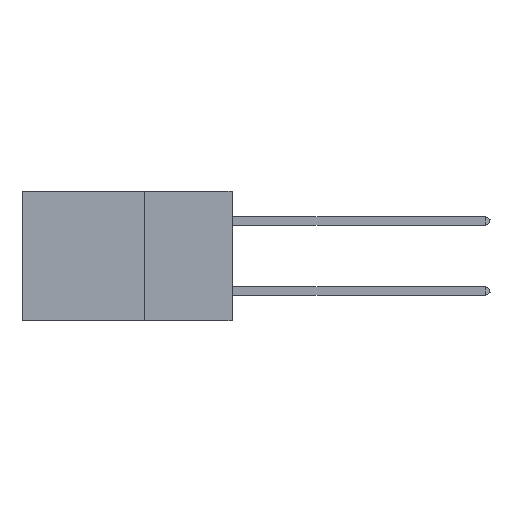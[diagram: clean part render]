
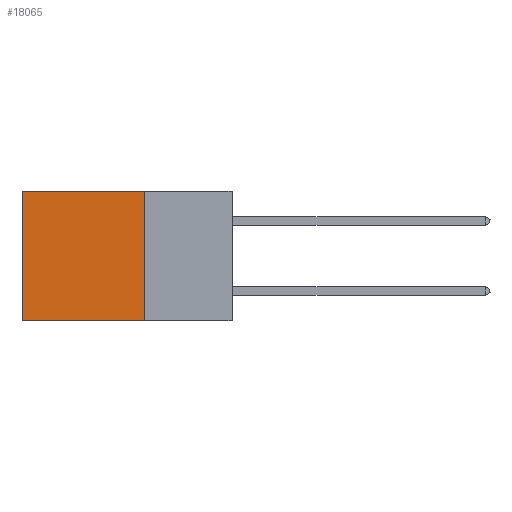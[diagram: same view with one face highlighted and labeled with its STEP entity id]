
A CAD part, left-side view. The second image highlights one B-rep face of the part: STEP entity #18065.
In plain terms, the highlighted planar face has unit normal (-1, 0, 0).
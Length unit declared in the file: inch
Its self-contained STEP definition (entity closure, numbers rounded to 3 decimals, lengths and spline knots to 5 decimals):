
#648 = CARTESIAN_POINT ( 'NONE',  ( 0.2875, 0.25, -0.37 ) ) ;
#2869 = CARTESIAN_POINT ( 'NONE',  ( 0.2875, 0.25, 0. ) ) ;
#2956 = CARTESIAN_POINT ( 'NONE',  ( 0.2875, 0.25, 0. ) ) ;
#3202 = ORIENTED_EDGE ( 'NONE', *, *, #32451, .T. ) ;
#3769 = VECTOR ( 'NONE', #14086, 39.37008 ) ;
#4389 = DIRECTION ( 'NONE',  ( 0., 1., 0. ) ) ;
#5817 = VECTOR ( 'NONE', #16964, 39.37008 ) ;
#6421 = AXIS2_PLACEMENT_3D ( 'NONE', #2956, #9793, #25693 ) ;
#7313 = CARTESIAN_POINT ( 'NONE',  ( 0.2875, 0.6, 0. ) ) ;
#7568 = CARTESIAN_POINT ( 'NONE',  ( 0.2875, 0.25, -0.37 ) ) ;
#8667 = VERTEX_POINT ( 'NONE', #12266 ) ;
#9659 = VERTEX_POINT ( 'NONE', #2869 ) ;
#9793 = DIRECTION ( 'NONE',  ( 1., 0., 0. ) ) ;
#10869 = CARTESIAN_POINT ( 'NONE',  ( 0.2875, 0.25, 0. ) ) ;
#11657 = VERTEX_POINT ( 'NONE', #648 ) ;
#12101 = LINE ( 'NONE', #7313, #41152 ) ;
#12266 = CARTESIAN_POINT ( 'NONE',  ( 0.2875, 0.6, -0.37 ) ) ;
#14086 = DIRECTION ( 'NONE',  ( 0., 0., -1. ) ) ;
#14724 = EDGE_CURVE ( 'NONE', #9659, #11657, #15796, .T. ) ;
#15796 = LINE ( 'NONE', #10869, #3769 ) ;
#16778 = CARTESIAN_POINT ( 'NONE',  ( 0.2875, 0.6, 0. ) ) ;
#16964 = DIRECTION ( 'NONE',  ( 0., 1., 0. ) ) ;
#17964 = ORIENTED_EDGE ( 'NONE', *, *, #38133, .T. ) ;
#18065 = ADVANCED_FACE ( 'NONE', ( #28497 ), #34841, .F. ) ;
#19539 = ORIENTED_EDGE ( 'NONE', *, *, #14724, .F. ) ;
#20559 = DIRECTION ( 'NONE',  ( 0., 0., -1. ) ) ;
#21649 = EDGE_LOOP ( 'NONE', ( #17964, #27028, #19539, #3202 ) ) ;
#24974 = EDGE_CURVE ( 'NONE', #11657, #8667, #34870, .T. ) ;
#25254 = VECTOR ( 'NONE', #4389, 39.37008 ) ;
#25693 = DIRECTION ( 'NONE',  ( 0., 0., -1. ) ) ;
#27028 = ORIENTED_EDGE ( 'NONE', *, *, #24974, .F. ) ;
#28497 = FACE_OUTER_BOUND ( 'NONE', #21649, .T. ) ;
#32451 = EDGE_CURVE ( 'NONE', #9659, #33656, #33809, .T. ) ;
#32928 = CARTESIAN_POINT ( 'NONE',  ( 0.2875, 0.25, 0. ) ) ;
#33656 = VERTEX_POINT ( 'NONE', #16778 ) ;
#33809 = LINE ( 'NONE', #32928, #25254 ) ;
#34841 = PLANE ( 'NONE',  #6421 ) ;
#34870 = LINE ( 'NONE', #7568, #5817 ) ;
#38133 = EDGE_CURVE ( 'NONE', #33656, #8667, #12101, .T. ) ;
#41152 = VECTOR ( 'NONE', #20559, 39.37008 ) ;
